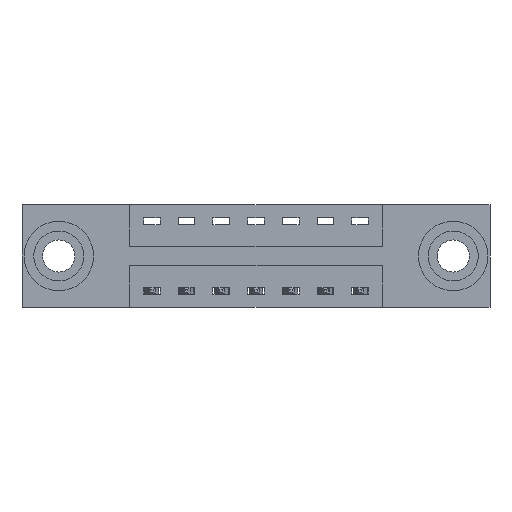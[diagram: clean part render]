
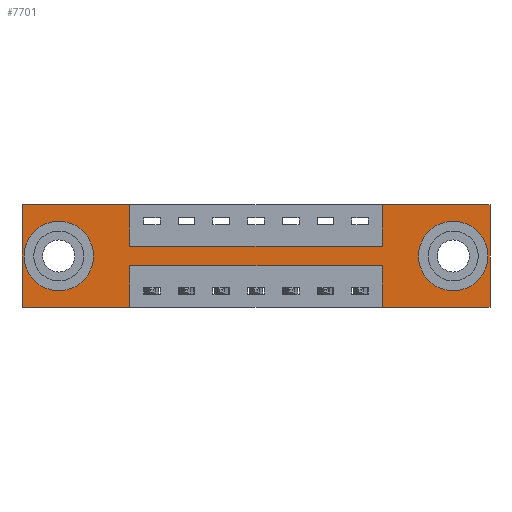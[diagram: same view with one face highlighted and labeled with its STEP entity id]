
A CAD part, front view. The second image highlights one B-rep face of the part: STEP entity #7701.
In plain terms, the highlighted planar face has unit normal (0, -1, 0).
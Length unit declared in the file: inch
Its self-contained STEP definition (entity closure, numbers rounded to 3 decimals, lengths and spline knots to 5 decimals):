
#139 = LINE ( 'NONE', #3286, #6637 ) ;
#146 = DIRECTION ( 'NONE',  ( 0., 0., -1. ) ) ;
#174 = DIRECTION ( 'NONE',  ( -1., 0., 0. ) ) ;
#335 = CARTESIAN_POINT ( 'NONE',  ( 1.2975, 0., -0.15 ) ) ;
#350 = CARTESIAN_POINT ( 'NONE',  ( 1.685, 0., 0. ) ) ;
#380 = VERTEX_POINT ( 'NONE', #5320 ) ;
#393 = EDGE_CURVE ( 'NONE', #7304, #1030, #8465, .T. ) ;
#398 = LINE ( 'NONE', #1943, #8083 ) ;
#503 = AXIS2_PLACEMENT_3D ( 'NONE', #5763, #5187, #8335 ) ;
#670 = ORIENTED_EDGE ( 'NONE', *, *, #3649, .T. ) ;
#700 = VERTEX_POINT ( 'NONE', #4914 ) ;
#716 = EDGE_CURVE ( 'NONE', #9759, #2429, #8316, .T. ) ;
#957 = VERTEX_POINT ( 'NONE', #9406 ) ;
#967 = CARTESIAN_POINT ( 'NONE',  ( 1.2975, 0., 0. ) ) ;
#1019 = DIRECTION ( 'NONE',  ( 1., 0., 0. ) ) ;
#1030 = VERTEX_POINT ( 'NONE', #335 ) ;
#1053 = ORIENTED_EDGE ( 'NONE', *, *, #8142, .F. ) ;
#1221 = CARTESIAN_POINT ( 'NONE',  ( 0., 0., 0. ) ) ;
#1271 = CIRCLE ( 'NONE', #7009, 0.078 ) ;
#1398 = CARTESIAN_POINT ( 'NONE',  ( 0., 0., -0.37 ) ) ;
#1431 = ORIENTED_EDGE ( 'NONE', *, *, #5538, .F. ) ;
#1543 = VECTOR ( 'NONE', #3125, 39.37008 ) ;
#1552 = CARTESIAN_POINT ( 'NONE',  ( 1.5525, 0., -0.185 ) ) ;
#1686 = CARTESIAN_POINT ( 'NONE',  ( 0.3875, 0., 0. ) ) ;
#1809 = DIRECTION ( 'NONE',  ( 0., 1., 0. ) ) ;
#1943 = CARTESIAN_POINT ( 'NONE',  ( 0., 0., 0. ) ) ;
#1968 = ORIENTED_EDGE ( 'NONE', *, *, #9866, .F. ) ;
#1969 = CARTESIAN_POINT ( 'NONE',  ( 0.3875, 0., -0.22 ) ) ;
#1992 = ORIENTED_EDGE ( 'NONE', *, *, #6011, .F. ) ;
#2017 = VECTOR ( 'NONE', #8870, 39.37008 ) ;
#2062 = CARTESIAN_POINT ( 'NONE',  ( 1.2975, 0., -0.37 ) ) ;
#2429 = VERTEX_POINT ( 'NONE', #3042 ) ;
#2564 = VERTEX_POINT ( 'NONE', #10117 ) ;
#2570 = LINE ( 'NONE', #5681, #2806 ) ;
#2614 = EDGE_CURVE ( 'NONE', #2429, #9759, #1271, .T. ) ;
#2806 = VECTOR ( 'NONE', #4830, 39.37008 ) ;
#2890 = ORIENTED_EDGE ( 'NONE', *, *, #8214, .F. ) ;
#2924 = DIRECTION ( 'NONE',  ( 0., -1., 0. ) ) ;
#2938 = VECTOR ( 'NONE', #146, 39.37008 ) ;
#3030 = CARTESIAN_POINT ( 'NONE',  ( 1.5525, 0., -0.263 ) ) ;
#3037 = LINE ( 'NONE', #10113, #8420 ) ;
#3042 = CARTESIAN_POINT ( 'NONE',  ( 1.5525, 0., -0.107 ) ) ;
#3086 = EDGE_CURVE ( 'NONE', #2564, #7304, #6315, .T. ) ;
#3125 = DIRECTION ( 'NONE',  ( 0., 0., 1. ) ) ;
#3148 = CIRCLE ( 'NONE', #503, 0.078 ) ;
#3176 = EDGE_CURVE ( 'NONE', #4247, #2564, #6670, .T. ) ;
#3240 = VERTEX_POINT ( 'NONE', #350 ) ;
#3286 = CARTESIAN_POINT ( 'NONE',  ( 1.2975, 0., 0. ) ) ;
#3381 = ORIENTED_EDGE ( 'NONE', *, *, #393, .F. ) ;
#3493 = ORIENTED_EDGE ( 'NONE', *, *, #3086, .F. ) ;
#3614 = DIRECTION ( 'NONE',  ( 0., 0., 1. ) ) ;
#3649 = EDGE_CURVE ( 'NONE', #9651, #5443, #6389, .T. ) ;
#3659 = EDGE_CURVE ( 'NONE', #957, #4824, #4334, .T. ) ;
#3685 = PLANE ( 'NONE',  #4655 ) ;
#3717 = CARTESIAN_POINT ( 'NONE',  ( 0.1325, 0., -0.185 ) ) ;
#3879 = AXIS2_PLACEMENT_3D ( 'NONE', #1552, #4751, #7107 ) ;
#3951 = EDGE_LOOP ( 'NONE', ( #3966, #7883 ) ) ;
#3966 = ORIENTED_EDGE ( 'NONE', *, *, #2614, .T. ) ;
#4153 = DIRECTION ( 'NONE',  ( 0., 0., 1. ) ) ;
#4247 = VERTEX_POINT ( 'NONE', #5576 ) ;
#4261 = VERTEX_POINT ( 'NONE', #967 ) ;
#4334 = LINE ( 'NONE', #7519, #9987 ) ;
#4348 = EDGE_CURVE ( 'NONE', #380, #4247, #2570, .T. ) ;
#4355 = DIRECTION ( 'NONE',  ( 1., 0., 0. ) ) ;
#4447 = CARTESIAN_POINT ( 'NONE',  ( 1.2975, 0., -0.22 ) ) ;
#4473 = VECTOR ( 'NONE', #174, 39.37008 ) ;
#4655 = AXIS2_PLACEMENT_3D ( 'NONE', #9940, #2924, #9178 ) ;
#4749 = EDGE_LOOP ( 'NONE', ( #5364, #1053, #1968, #10051, #2890, #1431, #9576, #3381, #3493, #7710, #6820, #1992 ) ) ;
#4751 = DIRECTION ( 'NONE',  ( 0., 1., 0. ) ) ;
#4791 = CARTESIAN_POINT ( 'NONE',  ( 1.5525, 0., -0.185 ) ) ;
#4824 = VERTEX_POINT ( 'NONE', #7486 ) ;
#4830 = DIRECTION ( 'NONE',  ( 0., 0., 1. ) ) ;
#4855 = VECTOR ( 'NONE', #7266, 39.37008 ) ;
#4914 = CARTESIAN_POINT ( 'NONE',  ( 1.2975, 0., -0.37 ) ) ;
#5045 = DIRECTION ( 'NONE',  ( 0., 1., 0. ) ) ;
#5049 = VERTEX_POINT ( 'NONE', #4447 ) ;
#5187 = DIRECTION ( 'NONE',  ( 0., 1., 0. ) ) ;
#5247 = LINE ( 'NONE', #1398, #7452 ) ;
#5320 = CARTESIAN_POINT ( 'NONE',  ( 0., 0., -0.37 ) ) ;
#5339 = EDGE_CURVE ( 'NONE', #5443, #9651, #3148, .T. ) ;
#5357 = CARTESIAN_POINT ( 'NONE',  ( 0.3875, 0., -0.15 ) ) ;
#5364 = ORIENTED_EDGE ( 'NONE', *, *, #3659, .F. ) ;
#5443 = VERTEX_POINT ( 'NONE', #7667 ) ;
#5538 = EDGE_CURVE ( 'NONE', #4261, #3240, #398, .T. ) ;
#5576 = CARTESIAN_POINT ( 'NONE',  ( 0., 0., 0. ) ) ;
#5654 = LINE ( 'NONE', #1969, #4473 ) ;
#5681 = CARTESIAN_POINT ( 'NONE',  ( 0., 0., 0. ) ) ;
#5724 = CARTESIAN_POINT ( 'NONE',  ( 1.685, 0., -0.37 ) ) ;
#5763 = CARTESIAN_POINT ( 'NONE',  ( 0.1325, 0., -0.185 ) ) ;
#5964 = DIRECTION ( 'NONE',  ( 0., 0., -1. ) ) ;
#5992 = FACE_BOUND ( 'NONE', #3951, .T. ) ;
#6011 = EDGE_CURVE ( 'NONE', #4824, #380, #5247, .T. ) ;
#6168 = DIRECTION ( 'NONE',  ( 0., 0., -1. ) ) ;
#6229 = AXIS2_PLACEMENT_3D ( 'NONE', #3717, #5045, #3614 ) ;
#6315 = LINE ( 'NONE', #1686, #2938 ) ;
#6389 = CIRCLE ( 'NONE', #6229, 0.078 ) ;
#6637 = VECTOR ( 'NONE', #4153, 39.37008 ) ;
#6670 = LINE ( 'NONE', #1221, #8357 ) ;
#6820 = ORIENTED_EDGE ( 'NONE', *, *, #4348, .F. ) ;
#6895 = CARTESIAN_POINT ( 'NONE',  ( 0.3875, 0., -0.15 ) ) ;
#7009 = AXIS2_PLACEMENT_3D ( 'NONE', #4791, #1809, #7249 ) ;
#7107 = DIRECTION ( 'NONE',  ( 0., 0., -1. ) ) ;
#7249 = DIRECTION ( 'NONE',  ( 0., 0., -1. ) ) ;
#7266 = DIRECTION ( 'NONE',  ( 1., 0., 0. ) ) ;
#7304 = VERTEX_POINT ( 'NONE', #6895 ) ;
#7449 = EDGE_LOOP ( 'NONE', ( #9095, #670 ) ) ;
#7452 = VECTOR ( 'NONE', #7479, 39.37008 ) ;
#7479 = DIRECTION ( 'NONE',  ( -1., 0., 0. ) ) ;
#7486 = CARTESIAN_POINT ( 'NONE',  ( 0.3875, 0., -0.37 ) ) ;
#7519 = CARTESIAN_POINT ( 'NONE',  ( 0.3875, 0., -0.37 ) ) ;
#7591 = FACE_BOUND ( 'NONE', #7449, .T. ) ;
#7667 = CARTESIAN_POINT ( 'NONE',  ( 0.1325, 0., -0.107 ) ) ;
#7701 = ADVANCED_FACE ( 'NONE', ( #5992, #7591, #9128 ), #3685, .T. ) ;
#7710 = ORIENTED_EDGE ( 'NONE', *, *, #3176, .F. ) ;
#7735 = EDGE_CURVE ( 'NONE', #9943, #700, #9745, .T. ) ;
#7883 = ORIENTED_EDGE ( 'NONE', *, *, #716, .T. ) ;
#8083 = VECTOR ( 'NONE', #4355, 39.37008 ) ;
#8142 = EDGE_CURVE ( 'NONE', #5049, #957, #5654, .T. ) ;
#8167 = CARTESIAN_POINT ( 'NONE',  ( 0., 0., -0.37 ) ) ;
#8214 = EDGE_CURVE ( 'NONE', #3240, #9943, #3037, .T. ) ;
#8316 = CIRCLE ( 'NONE', #3879, 0.078 ) ;
#8335 = DIRECTION ( 'NONE',  ( 0., 0., 1. ) ) ;
#8357 = VECTOR ( 'NONE', #1019, 39.37008 ) ;
#8420 = VECTOR ( 'NONE', #6168, 39.37008 ) ;
#8465 = LINE ( 'NONE', #5357, #4855 ) ;
#8870 = DIRECTION ( 'NONE',  ( -1., 0., 0. ) ) ;
#9095 = ORIENTED_EDGE ( 'NONE', *, *, #5339, .T. ) ;
#9128 = FACE_OUTER_BOUND ( 'NONE', #4749, .T. ) ;
#9178 = DIRECTION ( 'NONE',  ( 0., 0., -1. ) ) ;
#9289 = LINE ( 'NONE', #2062, #1543 ) ;
#9406 = CARTESIAN_POINT ( 'NONE',  ( 0.3875, 0., -0.22 ) ) ;
#9576 = ORIENTED_EDGE ( 'NONE', *, *, #10007, .F. ) ;
#9651 = VERTEX_POINT ( 'NONE', #9654 ) ;
#9654 = CARTESIAN_POINT ( 'NONE',  ( 0.1325, 0., -0.263 ) ) ;
#9745 = LINE ( 'NONE', #8167, #2017 ) ;
#9759 = VERTEX_POINT ( 'NONE', #3030 ) ;
#9866 = EDGE_CURVE ( 'NONE', #700, #5049, #9289, .T. ) ;
#9940 = CARTESIAN_POINT ( 'NONE',  ( 0., 0., -0.37 ) ) ;
#9943 = VERTEX_POINT ( 'NONE', #5724 ) ;
#9987 = VECTOR ( 'NONE', #5964, 39.37008 ) ;
#10007 = EDGE_CURVE ( 'NONE', #1030, #4261, #139, .T. ) ;
#10051 = ORIENTED_EDGE ( 'NONE', *, *, #7735, .F. ) ;
#10113 = CARTESIAN_POINT ( 'NONE',  ( 1.685, 0., 0. ) ) ;
#10117 = CARTESIAN_POINT ( 'NONE',  ( 0.3875, 0., 0. ) ) ;
